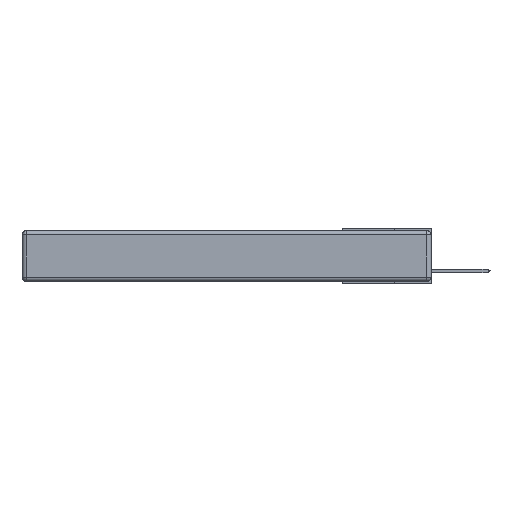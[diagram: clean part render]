
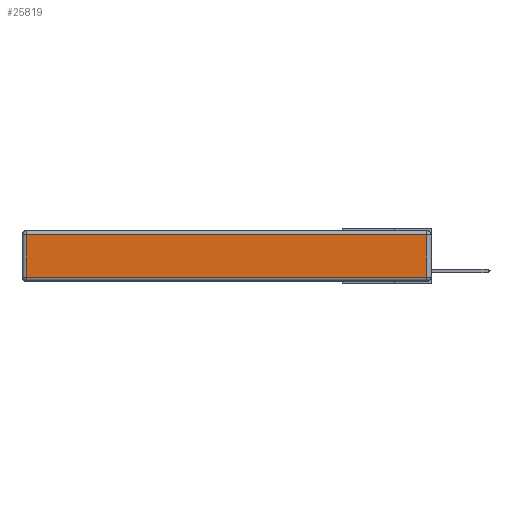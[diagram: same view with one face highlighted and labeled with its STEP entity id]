
A CAD part, left-side view. The second image highlights one B-rep face of the part: STEP entity #25819.
In plain terms, the highlighted planar face has unit normal (-1, 0, 0).
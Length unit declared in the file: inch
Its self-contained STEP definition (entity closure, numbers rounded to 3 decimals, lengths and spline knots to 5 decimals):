
#106 = VERTEX_POINT ( 'NONE', #32983 ) ;
#3218 = EDGE_CURVE ( 'NONE', #26369, #25131, #12357, .T. ) ;
#4678 = VECTOR ( 'NONE', #4758, 39.37008 ) ;
#4758 = DIRECTION ( 'NONE',  ( 0., 1., 0. ) ) ;
#6641 = DIRECTION ( 'NONE',  ( 0., 0., -1. ) ) ;
#6727 = LINE ( 'NONE', #10877, #33324 ) ;
#8539 = EDGE_CURVE ( 'NONE', #19901, #26369, #6727, .T. ) ;
#8971 = AXIS2_PLACEMENT_3D ( 'NONE', #23189, #15338, #15560 ) ;
#9030 = LINE ( 'NONE', #19551, #19476 ) ;
#10877 = CARTESIAN_POINT ( 'NONE',  ( 0., 0.03, -0.343 ) ) ;
#12278 = CARTESIAN_POINT ( 'NONE',  ( 0., 0.03, -0.03 ) ) ;
#12357 = LINE ( 'NONE', #28183, #4678 ) ;
#12409 = EDGE_LOOP ( 'NONE', ( #24635, #27587, #13087, #24055 ) ) ;
#13087 = ORIENTED_EDGE ( 'NONE', *, *, #3218, .T. ) ;
#13272 = LINE ( 'NONE', #14090, #23719 ) ;
#14090 = CARTESIAN_POINT ( 'NONE',  ( 0., 2.72, -0.343 ) ) ;
#15338 = DIRECTION ( 'NONE',  ( -1., 0., 0. ) ) ;
#15560 = DIRECTION ( 'NONE',  ( 0., 0., 1. ) ) ;
#19476 = VECTOR ( 'NONE', #32660, 39.37008 ) ;
#19551 = CARTESIAN_POINT ( 'NONE',  ( 0., 0., -0.313 ) ) ;
#19901 = VERTEX_POINT ( 'NONE', #26955 ) ;
#21222 = DIRECTION ( 'NONE',  ( 0., 0., 1. ) ) ;
#23189 = CARTESIAN_POINT ( 'NONE',  ( 0., 0., -0.343 ) ) ;
#23719 = VECTOR ( 'NONE', #6641, 39.37008 ) ;
#24055 = ORIENTED_EDGE ( 'NONE', *, *, #26127, .T. ) ;
#24635 = ORIENTED_EDGE ( 'NONE', *, *, #24944, .T. ) ;
#24944 = EDGE_CURVE ( 'NONE', #106, #19901, #9030, .T. ) ;
#25131 = VERTEX_POINT ( 'NONE', #26295 ) ;
#25819 = ADVANCED_FACE ( 'NONE', ( #25859 ), #28410, .T. ) ;
#25859 = FACE_OUTER_BOUND ( 'NONE', #12409, .T. ) ;
#26127 = EDGE_CURVE ( 'NONE', #25131, #106, #13272, .T. ) ;
#26295 = CARTESIAN_POINT ( 'NONE',  ( 0., 2.72, -0.03 ) ) ;
#26369 = VERTEX_POINT ( 'NONE', #12278 ) ;
#26955 = CARTESIAN_POINT ( 'NONE',  ( 0., 0.03, -0.313 ) ) ;
#27587 = ORIENTED_EDGE ( 'NONE', *, *, #8539, .T. ) ;
#28183 = CARTESIAN_POINT ( 'NONE',  ( 0., 2.75, -0.03 ) ) ;
#28410 = PLANE ( 'NONE',  #8971 ) ;
#32660 = DIRECTION ( 'NONE',  ( 0., -1., 0. ) ) ;
#32983 = CARTESIAN_POINT ( 'NONE',  ( 0., 2.72, -0.313 ) ) ;
#33324 = VECTOR ( 'NONE', #21222, 39.37008 ) ;
